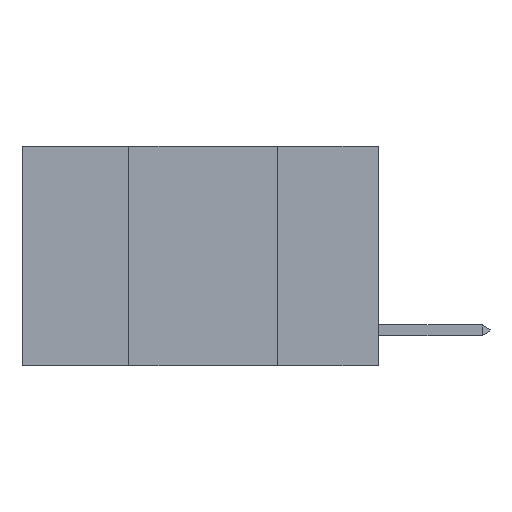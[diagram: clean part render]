
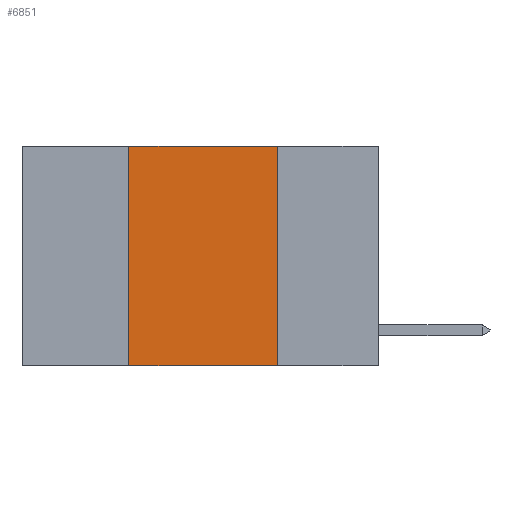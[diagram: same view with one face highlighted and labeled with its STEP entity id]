
A CAD part, left-side view. The second image highlights one B-rep face of the part: STEP entity #6851.
In plain terms, the highlighted planar face has unit normal (-1, 0, 0).
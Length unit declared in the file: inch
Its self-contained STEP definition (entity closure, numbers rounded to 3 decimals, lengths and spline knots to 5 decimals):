
#50 = CARTESIAN_POINT ( 'NONE',  ( 0., 0.42, -0.37 ) ) ;
#224 = CARTESIAN_POINT ( 'NONE',  ( 0., 0.17, -0.37 ) ) ;
#355 = FACE_OUTER_BOUND ( 'NONE', #17289, .T. ) ;
#962 = VECTOR ( 'NONE', #10562, 39.37008 ) ;
#3359 = LINE ( 'NONE', #10741, #962 ) ;
#3405 = DIRECTION ( 'NONE',  ( 1., 0., 0. ) ) ;
#4881 = DIRECTION ( 'NONE',  ( 0., 0., 1. ) ) ;
#5322 = VERTEX_POINT ( 'NONE', #17364 ) ;
#5354 = CARTESIAN_POINT ( 'NONE',  ( 0., 0.6, -0.37 ) ) ;
#5898 = ORIENTED_EDGE ( 'NONE', *, *, #9766, .F. ) ;
#6359 = CARTESIAN_POINT ( 'NONE',  ( 0., 0.42, 0. ) ) ;
#6405 = CARTESIAN_POINT ( 'NONE',  ( 0., 0.6, 0. ) ) ;
#6561 = DIRECTION ( 'NONE',  ( 0., 0., -1. ) ) ;
#6851 = ADVANCED_FACE ( 'NONE', ( #355 ), #16811, .F. ) ;
#7018 = VECTOR ( 'NONE', #10278, 39.37008 ) ;
#7139 = VECTOR ( 'NONE', #4881, 39.37008 ) ;
#7272 = AXIS2_PLACEMENT_3D ( 'NONE', #15122, #3405, #6561 ) ;
#7355 = ORIENTED_EDGE ( 'NONE', *, *, #19211, .T. ) ;
#7545 = VECTOR ( 'NONE', #9548, 39.37008 ) ;
#7719 = EDGE_CURVE ( 'NONE', #15025, #5322, #13770, .T. ) ;
#8108 = LINE ( 'NONE', #6359, #7139 ) ;
#9548 = DIRECTION ( 'NONE',  ( 0., -1., 0. ) ) ;
#9682 = VERTEX_POINT ( 'NONE', #50 ) ;
#9766 = EDGE_CURVE ( 'NONE', #9682, #15025, #8108, .T. ) ;
#10278 = DIRECTION ( 'NONE',  ( 0., -1., 0. ) ) ;
#10562 = DIRECTION ( 'NONE',  ( 0., 0., -1. ) ) ;
#10741 = CARTESIAN_POINT ( 'NONE',  ( 0., 0.17, 0. ) ) ;
#13641 = CARTESIAN_POINT ( 'NONE',  ( 0., 0.42, 0. ) ) ;
#13770 = LINE ( 'NONE', #6405, #7545 ) ;
#15025 = VERTEX_POINT ( 'NONE', #13641 ) ;
#15122 = CARTESIAN_POINT ( 'NONE',  ( 0., 0.6, 0. ) ) ;
#15201 = ORIENTED_EDGE ( 'NONE', *, *, #7719, .F. ) ;
#15435 = ORIENTED_EDGE ( 'NONE', *, *, #17207, .F. ) ;
#16811 = PLANE ( 'NONE',  #7272 ) ;
#17207 = EDGE_CURVE ( 'NONE', #5322, #18840, #3359, .T. ) ;
#17289 = EDGE_LOOP ( 'NONE', ( #15435, #15201, #5898, #7355 ) ) ;
#17364 = CARTESIAN_POINT ( 'NONE',  ( 0., 0.17, 0. ) ) ;
#18840 = VERTEX_POINT ( 'NONE', #224 ) ;
#19205 = LINE ( 'NONE', #5354, #7018 ) ;
#19211 = EDGE_CURVE ( 'NONE', #9682, #18840, #19205, .T. ) ;
